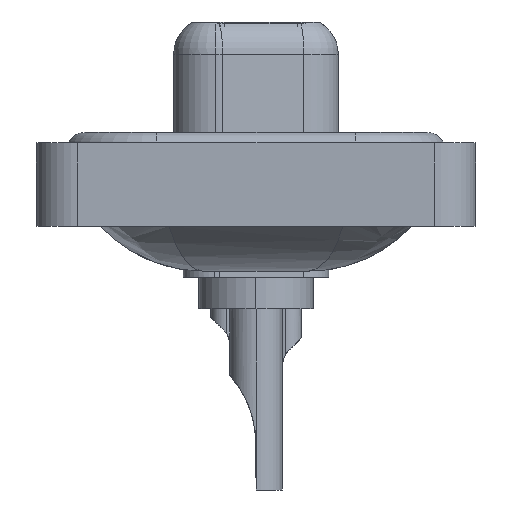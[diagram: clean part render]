
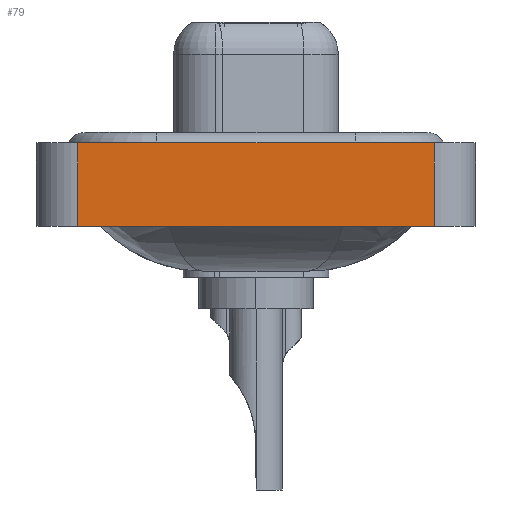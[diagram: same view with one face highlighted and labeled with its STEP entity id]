
A CAD part, left-side view. The second image highlights one B-rep face of the part: STEP entity #79.
In plain terms, the highlighted planar face has unit normal (-1, 0, 0).
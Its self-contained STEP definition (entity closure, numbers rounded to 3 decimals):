
#79 = ADVANCED_FACE ( 'NONE', ( #21211 ), #22689, .T. ) ;
#914 = DIRECTION ( 'NONE',  ( 0., 0., 1. ) ) ;
#1391 = EDGE_CURVE ( 'NONE', #8168, #20811, #2016, .T. ) ;
#2016 = LINE ( 'NONE', #10473, #20220 ) ;
#2031 = VECTOR ( 'NONE', #20894, 1000. ) ;
#2788 = EDGE_CURVE ( 'NONE', #4132, #12882, #14197, .T. ) ;
#3530 = CARTESIAN_POINT ( 'NONE',  ( -7.35, -8.55, 0.4 ) ) ;
#4132 = VERTEX_POINT ( 'NONE', #8021 ) ;
#4602 = ORIENTED_EDGE ( 'NONE', *, *, #2788, .F. ) ;
#4719 = EDGE_CURVE ( 'NONE', #12882, #20811, #9664, .T. ) ;
#5310 = CARTESIAN_POINT ( 'NONE',  ( -7.35, -8.55, -3.6 ) ) ;
#5521 = ORIENTED_EDGE ( 'NONE', *, *, #6103, .T. ) ;
#6005 = DIRECTION ( 'NONE',  ( 0., 0., 1. ) ) ;
#6103 = EDGE_CURVE ( 'NONE', #4132, #8168, #10716, .T. ) ;
#6370 = ORIENTED_EDGE ( 'NONE', *, *, #1391, .T. ) ;
#7800 = CARTESIAN_POINT ( 'NONE',  ( -7.35, 8.55, 0.4 ) ) ;
#8021 = CARTESIAN_POINT ( 'NONE',  ( -7.35, 8.55, -3.6 ) ) ;
#8168 = VERTEX_POINT ( 'NONE', #5310 ) ;
#8805 = EDGE_LOOP ( 'NONE', ( #6370, #16359, #4602, #5521 ) ) ;
#8842 = VECTOR ( 'NONE', #16838, 1000. ) ;
#9664 = LINE ( 'NONE', #11896, #2031 ) ;
#10473 = CARTESIAN_POINT ( 'NONE',  ( -7.35, -8.55, -3.6 ) ) ;
#10716 = LINE ( 'NONE', #16700, #8842 ) ;
#11470 = AXIS2_PLACEMENT_3D ( 'NONE', #11709, #22827, #6005 ) ;
#11709 = CARTESIAN_POINT ( 'NONE',  ( -7.35, -8.55, -3.6 ) ) ;
#11896 = CARTESIAN_POINT ( 'NONE',  ( -7.35, -8.55, 0.4 ) ) ;
#11964 = DIRECTION ( 'NONE',  ( 0., 0., 1. ) ) ;
#12882 = VERTEX_POINT ( 'NONE', #7800 ) ;
#14197 = LINE ( 'NONE', #19696, #16369 ) ;
#16359 = ORIENTED_EDGE ( 'NONE', *, *, #4719, .F. ) ;
#16369 = VECTOR ( 'NONE', #11964, 1000. ) ;
#16700 = CARTESIAN_POINT ( 'NONE',  ( -7.35, -8.55, -3.6 ) ) ;
#16838 = DIRECTION ( 'NONE',  ( 0., -1., 0. ) ) ;
#19696 = CARTESIAN_POINT ( 'NONE',  ( -7.35, 8.55, -3.6 ) ) ;
#20220 = VECTOR ( 'NONE', #914, 1000. ) ;
#20811 = VERTEX_POINT ( 'NONE', #3530 ) ;
#20894 = DIRECTION ( 'NONE',  ( 0., -1., 0. ) ) ;
#21211 = FACE_OUTER_BOUND ( 'NONE', #8805, .T. ) ;
#22689 = PLANE ( 'NONE',  #11470 ) ;
#22827 = DIRECTION ( 'NONE',  ( -1., 0., 0. ) ) ;
